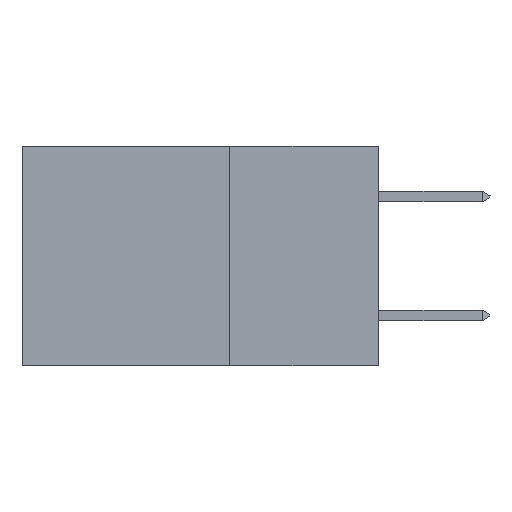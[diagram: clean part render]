
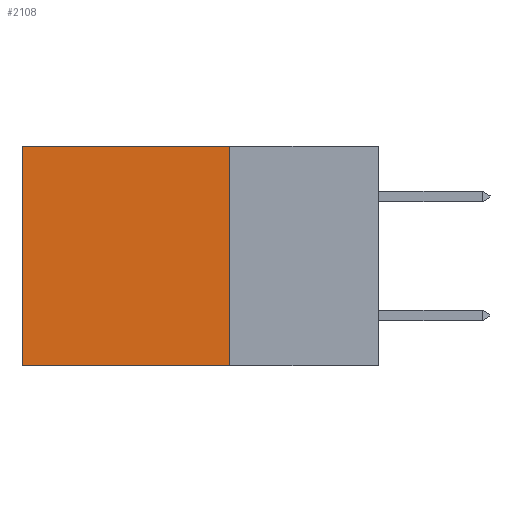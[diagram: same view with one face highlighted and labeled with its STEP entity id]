
A CAD part, left-side view. The second image highlights one B-rep face of the part: STEP entity #2108.
In plain terms, the highlighted planar face has unit normal (-1, 0, 0).
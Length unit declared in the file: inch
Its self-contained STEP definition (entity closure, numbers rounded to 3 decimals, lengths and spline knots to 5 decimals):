
#120 = PLANE ( 'NONE',  #8529 ) ;
#412 = DIRECTION ( 'NONE',  ( 0., 0., -1. ) ) ;
#1532 = CARTESIAN_POINT ( 'NONE',  ( 0.2615, 0.25, 0. ) ) ;
#2029 = VECTOR ( 'NONE', #412, 39.37008 ) ;
#2108 = ADVANCED_FACE ( 'NONE', ( #18196 ), #120, .F. ) ;
#3186 = DIRECTION ( 'NONE',  ( 0., 1., 0. ) ) ;
#3927 = VERTEX_POINT ( 'NONE', #4953 ) ;
#4691 = ORIENTED_EDGE ( 'NONE', *, *, #20653, .F. ) ;
#4953 = CARTESIAN_POINT ( 'NONE',  ( 0.2615, 0.6, 0. ) ) ;
#5576 = CARTESIAN_POINT ( 'NONE',  ( 0.2615, 0.25, -0.37 ) ) ;
#5627 = CARTESIAN_POINT ( 'NONE',  ( 0.2615, 0.25, -0.37 ) ) ;
#6490 = ORIENTED_EDGE ( 'NONE', *, *, #10753, .T. ) ;
#6833 = DIRECTION ( 'NONE',  ( 1., 0., 0. ) ) ;
#6925 = CARTESIAN_POINT ( 'NONE',  ( 0.2615, 0.6, -0.37 ) ) ;
#6995 = EDGE_CURVE ( 'NONE', #3927, #17984, #14300, .T. ) ;
#8051 = VERTEX_POINT ( 'NONE', #12119 ) ;
#8115 = ORIENTED_EDGE ( 'NONE', *, *, #6995, .T. ) ;
#8529 = AXIS2_PLACEMENT_3D ( 'NONE', #15015, #6833, #16590 ) ;
#10753 = EDGE_CURVE ( 'NONE', #8051, #3927, #14819, .T. ) ;
#12119 = CARTESIAN_POINT ( 'NONE',  ( 0.2615, 0.25, 0. ) ) ;
#12797 = VECTOR ( 'NONE', #3186, 39.37008 ) ;
#13271 = VECTOR ( 'NONE', #20983, 39.37008 ) ;
#14140 = VECTOR ( 'NONE', #18188, 39.37008 ) ;
#14300 = LINE ( 'NONE', #6925, #14140 ) ;
#14734 = CARTESIAN_POINT ( 'NONE',  ( 0.2615, 0.6, -0.37 ) ) ;
#14819 = LINE ( 'NONE', #1532, #13271 ) ;
#14857 = ORIENTED_EDGE ( 'NONE', *, *, #15283, .F. ) ;
#15015 = CARTESIAN_POINT ( 'NONE',  ( 0.2615, 0.25, -0.37 ) ) ;
#15283 = EDGE_CURVE ( 'NONE', #8051, #16342, #16769, .T. ) ;
#16034 = LINE ( 'NONE', #20916, #12797 ) ;
#16342 = VERTEX_POINT ( 'NONE', #5576 ) ;
#16590 = DIRECTION ( 'NONE',  ( 0., 0., -1. ) ) ;
#16769 = LINE ( 'NONE', #5627, #2029 ) ;
#17984 = VERTEX_POINT ( 'NONE', #14734 ) ;
#18188 = DIRECTION ( 'NONE',  ( 0., 0., -1. ) ) ;
#18196 = FACE_OUTER_BOUND ( 'NONE', #20191, .T. ) ;
#20191 = EDGE_LOOP ( 'NONE', ( #8115, #4691, #14857, #6490 ) ) ;
#20653 = EDGE_CURVE ( 'NONE', #16342, #17984, #16034, .T. ) ;
#20916 = CARTESIAN_POINT ( 'NONE',  ( 0.2615, 0.25, -0.37 ) ) ;
#20983 = DIRECTION ( 'NONE',  ( 0., 1., 0. ) ) ;
